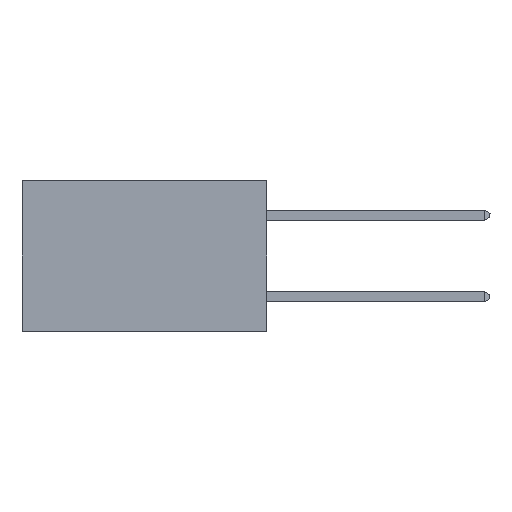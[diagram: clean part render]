
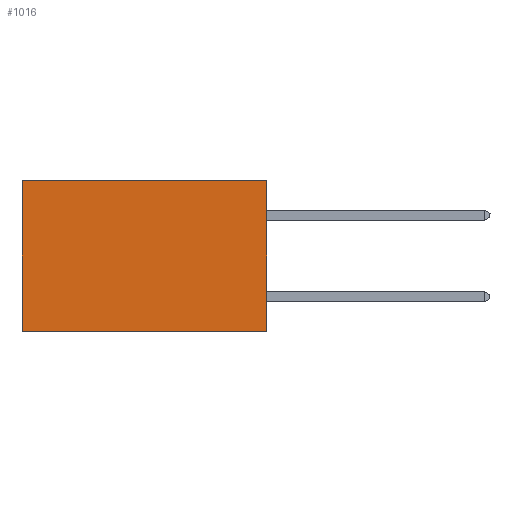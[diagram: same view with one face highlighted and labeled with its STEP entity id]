
A CAD part, left-side view. The second image highlights one B-rep face of the part: STEP entity #1016.
In plain terms, the highlighted planar face has unit normal (-1, 0, 0).
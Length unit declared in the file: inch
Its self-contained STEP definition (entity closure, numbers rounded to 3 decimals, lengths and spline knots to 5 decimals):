
#22 = DIRECTION ( 'NONE',  ( 0., 1., 0. ) ) ;
#118 = VECTOR ( 'NONE', #22, 39.37008 ) ;
#132 = EDGE_CURVE ( 'NONE', #10684, #14762, #15332, .T. ) ;
#809 = EDGE_CURVE ( 'NONE', #12440, #14762, #17214, .T. ) ;
#1016 = ADVANCED_FACE ( 'NONE', ( #12407 ), #18386, .F. ) ;
#1165 = ORIENTED_EDGE ( 'NONE', *, *, #18486, .T. ) ;
#1647 = DIRECTION ( 'NONE',  ( 0., 0., -1. ) ) ;
#1675 = EDGE_CURVE ( 'NONE', #16789, #10684, #17409, .T. ) ;
#2256 = ORIENTED_EDGE ( 'NONE', *, *, #1675, .F. ) ;
#3357 = VECTOR ( 'NONE', #6909, 39.37008 ) ;
#3951 = AXIS2_PLACEMENT_3D ( 'NONE', #12320, #18264, #1647 ) ;
#4612 = DIRECTION ( 'NONE',  ( 0., 1., 0. ) ) ;
#4813 = LINE ( 'NONE', #15128, #118 ) ;
#5442 = CARTESIAN_POINT ( 'NONE',  ( 0.2875, 0., 0. ) ) ;
#6766 = CARTESIAN_POINT ( 'NONE',  ( 0.2875, 0.6, -0.37 ) ) ;
#6909 = DIRECTION ( 'NONE',  ( 0., 0., -1. ) ) ;
#7595 = CARTESIAN_POINT ( 'NONE',  ( 0.2875, 0., -0.37 ) ) ;
#8631 = DIRECTION ( 'NONE',  ( 0., 0., -1. ) ) ;
#10684 = VERTEX_POINT ( 'NONE', #18164 ) ;
#11070 = EDGE_LOOP ( 'NONE', ( #12876, #18936, #2256, #1165 ) ) ;
#11768 = CARTESIAN_POINT ( 'NONE',  ( 0.2875, 0.6, 0. ) ) ;
#12320 = CARTESIAN_POINT ( 'NONE',  ( 0.2875, 0., 0. ) ) ;
#12407 = FACE_OUTER_BOUND ( 'NONE', #11070, .T. ) ;
#12440 = VERTEX_POINT ( 'NONE', #11768 ) ;
#12685 = VECTOR ( 'NONE', #8631, 39.37008 ) ;
#12783 = CARTESIAN_POINT ( 'NONE',  ( 0.2875, 0., 0. ) ) ;
#12876 = ORIENTED_EDGE ( 'NONE', *, *, #809, .T. ) ;
#13296 = CARTESIAN_POINT ( 'NONE',  ( 0.2875, 0.6, 0. ) ) ;
#14762 = VERTEX_POINT ( 'NONE', #6766 ) ;
#15128 = CARTESIAN_POINT ( 'NONE',  ( 0.2875, 0., 0. ) ) ;
#15332 = LINE ( 'NONE', #7595, #16762 ) ;
#16762 = VECTOR ( 'NONE', #4612, 39.37008 ) ;
#16789 = VERTEX_POINT ( 'NONE', #12783 ) ;
#17214 = LINE ( 'NONE', #13296, #12685 ) ;
#17409 = LINE ( 'NONE', #5442, #3357 ) ;
#18164 = CARTESIAN_POINT ( 'NONE',  ( 0.2875, 0., -0.37 ) ) ;
#18264 = DIRECTION ( 'NONE',  ( 1., 0., 0. ) ) ;
#18386 = PLANE ( 'NONE',  #3951 ) ;
#18486 = EDGE_CURVE ( 'NONE', #16789, #12440, #4813, .T. ) ;
#18936 = ORIENTED_EDGE ( 'NONE', *, *, #132, .F. ) ;
